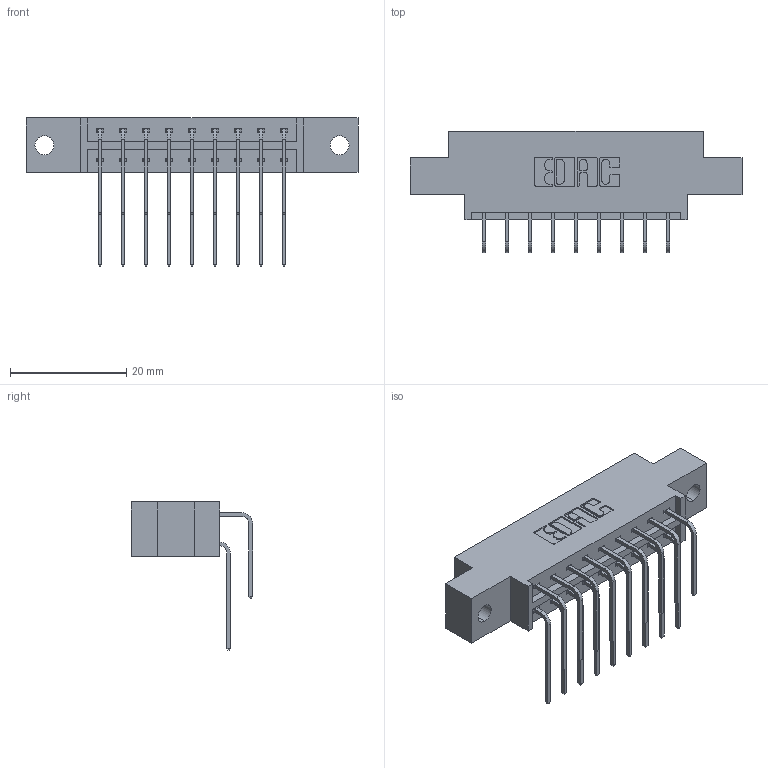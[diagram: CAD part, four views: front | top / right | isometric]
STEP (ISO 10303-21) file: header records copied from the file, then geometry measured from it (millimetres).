
FILE_DESCRIPTION (( 'STEP AP203' ), '1' );
FILE_NAME ('333-018-559-802.STEP', '2019-08-09T14:25:43', ( '' ), ( '' ), 'SwSTEP 2.0', 'SolidWorks 2016', '' );
FILE_SCHEMA (( 'CONFIG_CONTROL_DESIGN' ));
Length unit declared in the file: inch
Products named in the file (4): 345-292-001_558 559 Tail - 1; 333 Part_Offset - .128 Dia; 345-292-001_559 Tail - 2; 333-018-559-802
Assembly tree (19 placements, depth 2):
  333-018-559-802
    333 Part_Offset - .128 Dia
    345-292-001_558 559 Tail - 1  x9
    345-292-001_559 Tail - 2  x9
Bounding box: 57.2 x 20.9 x 25.53 mm (x, y, z)
Volume: 5370.6 mm3; surface area: 6459.5 mm2
Topology: 19 solids, 19 shells, 1090 faces, 3221 edges, 2122 vertices
Faces by surface type: plane 758, cylinder 332
Entity records: 11977 total; most frequent: CARTESIAN_POINT 2077, ORIENTED_EDGE 1962, DIRECTION 1813, EDGE_CURVE 981, VECTOR 813, LINE 813, VERTEX_POINT 650, AXIS2_PLACEMENT_3D 500
